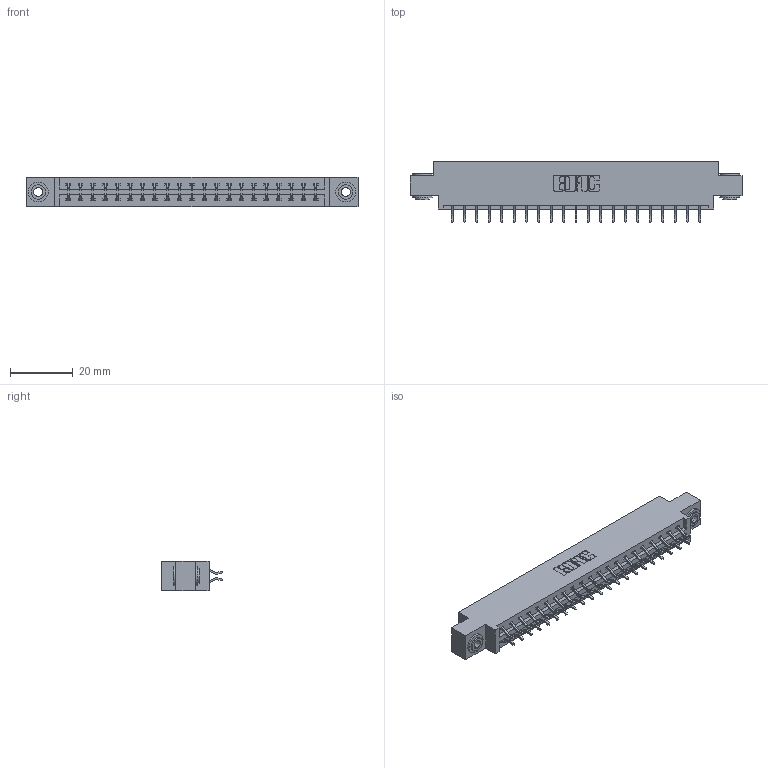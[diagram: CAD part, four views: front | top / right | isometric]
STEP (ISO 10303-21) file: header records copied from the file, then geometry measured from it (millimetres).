
FILE_DESCRIPTION (( 'STEP AP203' ), '1' );
FILE_NAME ('337-042-556-803.STEP', '2019-10-11T13:04:02', ( '' ), ( '' ), 'SwSTEP 2.0', 'SolidWorks 2016', '' );
FILE_SCHEMA (( 'CONFIG_CONTROL_DESIGN' ));
Length unit declared in the file: inch
Products named in the file (4): 337-042-556-803; 345-250-002_345-250-002-102; 345-292-001_556 Tail; 337 Part_0.170 Offset - 0.156 Dia-TH
Assembly tree (45 placements, depth 2):
  337-042-556-803
    337 Part_0.170 Offset - 0.156 Dia-TH
    345-292-001_556 Tail  x42
    345-250-002_345-250-002-102  x2
Bounding box: 106.22 x 19.57 x 9.4 mm (x, y, z)
Volume: 10815.3 mm3; surface area: 12310.6 mm2
Topology: 45 solids, 45 shells, 2676 faces, 7917 edges, 5218 vertices
Faces by surface type: plane 1848, cylinder 820, cone 8
Entity records: 20000 total; most frequent: CARTESIAN_POINT 3377, ORIENTED_EDGE 3294, DIRECTION 2933, EDGE_CURVE 1647, VECTOR 1487, LINE 1487, VERTEX_POINT 1094, AXIS2_PLACEMENT_3D 723
